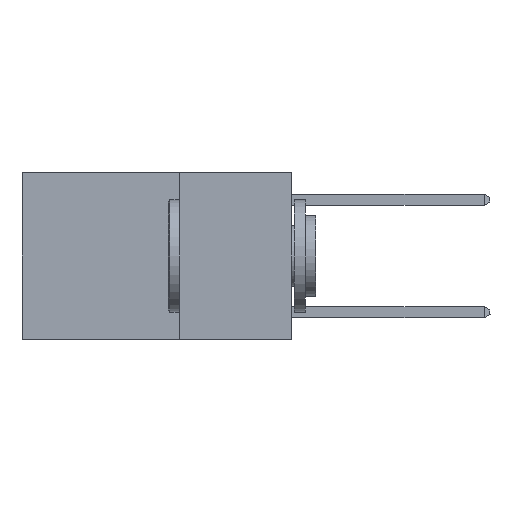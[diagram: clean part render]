
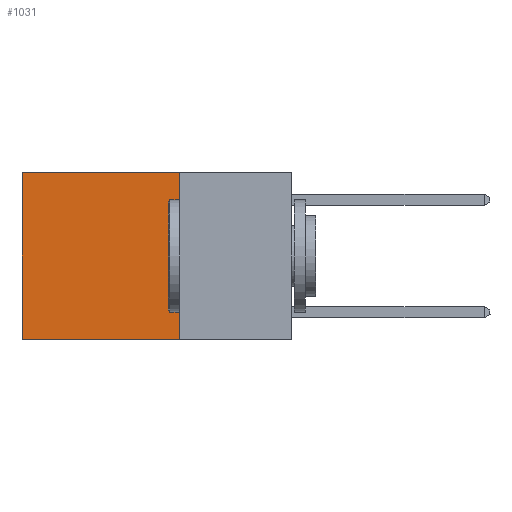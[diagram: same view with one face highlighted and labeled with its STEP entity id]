
A CAD part, left-side view. The second image highlights one B-rep face of the part: STEP entity #1031.
In plain terms, the highlighted planar face has unit normal (-1, 0, 0).
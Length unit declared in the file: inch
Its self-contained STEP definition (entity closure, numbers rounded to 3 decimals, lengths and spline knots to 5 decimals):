
#49 = VECTOR ( 'NONE', #8414, 39.37008 ) ;
#261 = CARTESIAN_POINT ( 'NONE',  ( 0.2625, 0.6, 0. ) ) ;
#511 = ORIENTED_EDGE ( 'NONE', *, *, #6129, .T. ) ;
#634 = DIRECTION ( 'NONE',  ( 0., 0., -1. ) ) ;
#825 = LINE ( 'NONE', #261, #4352 ) ;
#861 = CARTESIAN_POINT ( 'NONE',  ( 0.2625, 0.25, -0.37 ) ) ;
#1031 = ADVANCED_FACE ( 'NONE', ( #1960 ), #8489, .F. ) ;
#1139 = EDGE_LOOP ( 'NONE', ( #5690, #1368, #8235, #511 ) ) ;
#1269 = VECTOR ( 'NONE', #7566, 39.37008 ) ;
#1368 = ORIENTED_EDGE ( 'NONE', *, *, #2020, .F. ) ;
#1372 = LINE ( 'NONE', #4266, #2805 ) ;
#1960 = FACE_OUTER_BOUND ( 'NONE', #1139, .T. ) ;
#2020 = EDGE_CURVE ( 'NONE', #6284, #8837, #1372, .T. ) ;
#2773 = LINE ( 'NONE', #6315, #49 ) ;
#2805 = VECTOR ( 'NONE', #4917, 39.37008 ) ;
#2937 = CARTESIAN_POINT ( 'NONE',  ( 0.2625, 0.6, -0.37 ) ) ;
#2994 = EDGE_CURVE ( 'NONE', #3004, #8837, #825, .T. ) ;
#3004 = VERTEX_POINT ( 'NONE', #8860 ) ;
#3257 = CARTESIAN_POINT ( 'NONE',  ( 0.2625, 0.25, 0. ) ) ;
#4266 = CARTESIAN_POINT ( 'NONE',  ( 0.2625, 0.25, -0.37 ) ) ;
#4352 = VECTOR ( 'NONE', #5961, 39.37008 ) ;
#4860 = AXIS2_PLACEMENT_3D ( 'NONE', #7713, #5582, #634 ) ;
#4917 = DIRECTION ( 'NONE',  ( 0., 1., 0. ) ) ;
#5035 = EDGE_CURVE ( 'NONE', #9305, #6284, #2773, .T. ) ;
#5582 = DIRECTION ( 'NONE',  ( 1., 0., 0. ) ) ;
#5690 = ORIENTED_EDGE ( 'NONE', *, *, #2994, .T. ) ;
#5961 = DIRECTION ( 'NONE',  ( 0., 0., -1. ) ) ;
#6129 = EDGE_CURVE ( 'NONE', #9305, #3004, #6138, .T. ) ;
#6138 = LINE ( 'NONE', #6809, #1269 ) ;
#6284 = VERTEX_POINT ( 'NONE', #861 ) ;
#6315 = CARTESIAN_POINT ( 'NONE',  ( 0.2625, 0.25, 0. ) ) ;
#6809 = CARTESIAN_POINT ( 'NONE',  ( 0.2625, 0.25, 0. ) ) ;
#7566 = DIRECTION ( 'NONE',  ( 0., 1., 0. ) ) ;
#7713 = CARTESIAN_POINT ( 'NONE',  ( 0.2625, 0.25, 0. ) ) ;
#8235 = ORIENTED_EDGE ( 'NONE', *, *, #5035, .F. ) ;
#8414 = DIRECTION ( 'NONE',  ( 0., 0., -1. ) ) ;
#8489 = PLANE ( 'NONE',  #4860 ) ;
#8837 = VERTEX_POINT ( 'NONE', #2937 ) ;
#8860 = CARTESIAN_POINT ( 'NONE',  ( 0.2625, 0.6, 0. ) ) ;
#9305 = VERTEX_POINT ( 'NONE', #3257 ) ;
